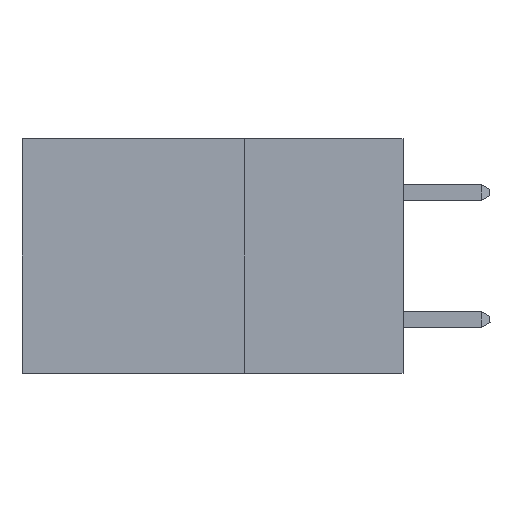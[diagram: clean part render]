
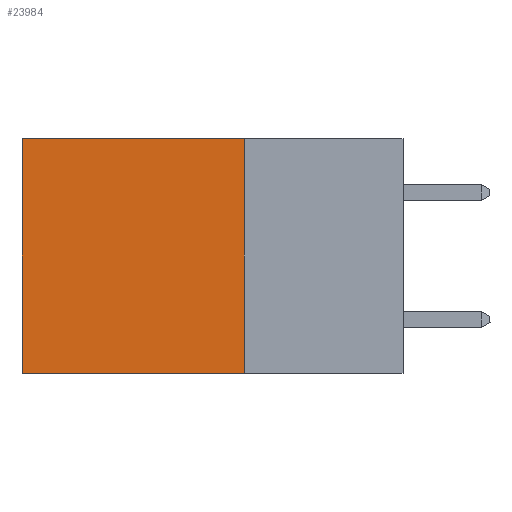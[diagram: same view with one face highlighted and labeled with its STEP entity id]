
A CAD part, left-side view. The second image highlights one B-rep face of the part: STEP entity #23984.
In plain terms, the highlighted planar face has unit normal (-1, 0, 0).
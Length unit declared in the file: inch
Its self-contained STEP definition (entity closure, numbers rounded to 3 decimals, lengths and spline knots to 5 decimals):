
#297 = ORIENTED_EDGE ( 'NONE', *, *, #14517, .T. ) ;
#1244 = EDGE_CURVE ( 'NONE', #7206, #15439, #10484, .T. ) ;
#1471 = DIRECTION ( 'NONE',  ( 0., 0., -1. ) ) ;
#1607 = DIRECTION ( 'NONE',  ( 0., 0., -1. ) ) ;
#3787 = CARTESIAN_POINT ( 'NONE',  ( 0.2875, 0.6, 0. ) ) ;
#5535 = PLANE ( 'NONE',  #8791 ) ;
#6084 = VERTEX_POINT ( 'NONE', #16398 ) ;
#6281 = CARTESIAN_POINT ( 'NONE',  ( 0.2875, 0.25, -0.37 ) ) ;
#6505 = EDGE_CURVE ( 'NONE', #6084, #7206, #19078, .T. ) ;
#7120 = CARTESIAN_POINT ( 'NONE',  ( 0.2875, 0.6, 0. ) ) ;
#7131 = DIRECTION ( 'NONE',  ( 0., 1., 0. ) ) ;
#7206 = VERTEX_POINT ( 'NONE', #12021 ) ;
#7435 = DIRECTION ( 'NONE',  ( 0., 1., 0. ) ) ;
#8791 = AXIS2_PLACEMENT_3D ( 'NONE', #19750, #23865, #1471 ) ;
#9582 = VECTOR ( 'NONE', #23507, 39.37008 ) ;
#10484 = LINE ( 'NONE', #6281, #15543 ) ;
#11516 = CARTESIAN_POINT ( 'NONE',  ( 0.2875, 0.25, 0. ) ) ;
#12021 = CARTESIAN_POINT ( 'NONE',  ( 0.2875, 0.25, -0.37 ) ) ;
#12271 = VERTEX_POINT ( 'NONE', #7120 ) ;
#12283 = ORIENTED_EDGE ( 'NONE', *, *, #1244, .F. ) ;
#13390 = VECTOR ( 'NONE', #7435, 39.37008 ) ;
#14517 = EDGE_CURVE ( 'NONE', #12271, #15439, #20665, .T. ) ;
#15439 = VERTEX_POINT ( 'NONE', #23236 ) ;
#15543 = VECTOR ( 'NONE', #7131, 39.37008 ) ;
#16086 = EDGE_LOOP ( 'NONE', ( #297, #12283, #18734, #17991 ) ) ;
#16398 = CARTESIAN_POINT ( 'NONE',  ( 0.2875, 0.25, 0. ) ) ;
#17449 = VECTOR ( 'NONE', #1607, 39.37008 ) ;
#17991 = ORIENTED_EDGE ( 'NONE', *, *, #24987, .T. ) ;
#18734 = ORIENTED_EDGE ( 'NONE', *, *, #6505, .F. ) ;
#18910 = CARTESIAN_POINT ( 'NONE',  ( 0.2875, 0.25, 0. ) ) ;
#19078 = LINE ( 'NONE', #18910, #9582 ) ;
#19750 = CARTESIAN_POINT ( 'NONE',  ( 0.2875, 0.25, 0. ) ) ;
#20665 = LINE ( 'NONE', #3787, #17449 ) ;
#21695 = LINE ( 'NONE', #11516, #13390 ) ;
#23236 = CARTESIAN_POINT ( 'NONE',  ( 0.2875, 0.6, -0.37 ) ) ;
#23507 = DIRECTION ( 'NONE',  ( 0., 0., -1. ) ) ;
#23865 = DIRECTION ( 'NONE',  ( 1., 0., 0. ) ) ;
#23984 = ADVANCED_FACE ( 'NONE', ( #26240 ), #5535, .F. ) ;
#24987 = EDGE_CURVE ( 'NONE', #6084, #12271, #21695, .T. ) ;
#26240 = FACE_OUTER_BOUND ( 'NONE', #16086, .T. ) ;
